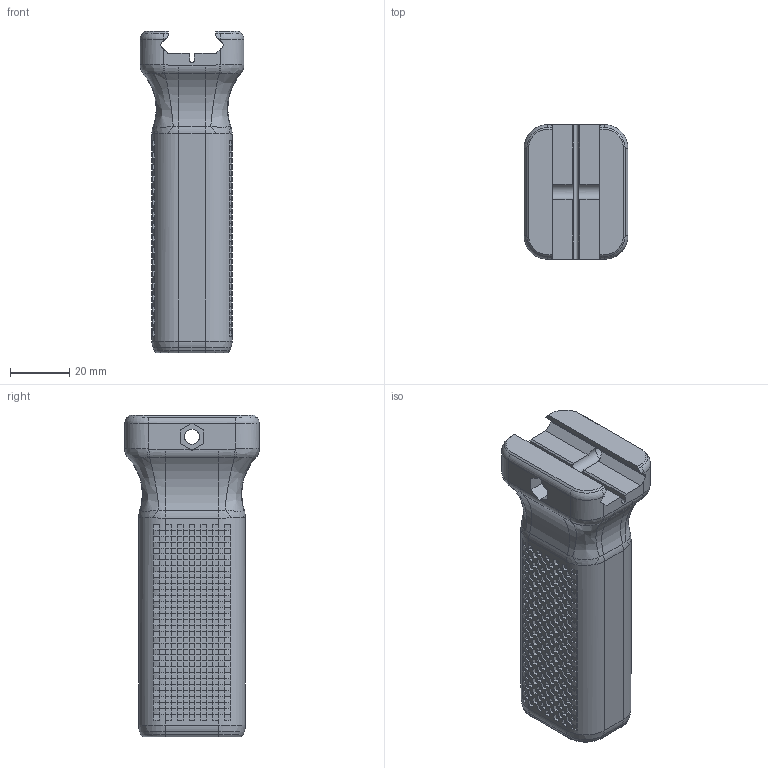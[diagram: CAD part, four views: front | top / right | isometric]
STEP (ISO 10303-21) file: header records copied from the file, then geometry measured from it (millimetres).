
FILE_DESCRIPTION(/* description */ (''),/* implementation_level */ '2;1');
FILE_NAME(/* name */ 'Checkered Model.step',/* time_stamp */ '2021-05-21T12:31:54-04:00',/* author */ (''),/* organization */ (''),/* preprocessor_version */ 'ST-DEVELOPER v18.1',/* originating_system */ 'Autodesk Translation Framework v10.6.0.1341',/* authorisation */ '');
FILE_SCHEMA (('AUTOMOTIVE_DESIGN { 1 0 10303 214 3 1 1 }'));
Products named in the file (1): Checkered Model
Bounding box: 35 x 45.3 x 108.12 mm (x, y, z)
Volume: 55236.5 mm3; surface area: 26486.5 mm2
Topology: 1 solids, 1 shells, 3015 faces, 6425 edges, 2646 vertices
Faces by surface type: plane 2725, cylinder 174, bspline 84, torus 20, cone 12
Full cylindrical faces by diameter (mm): 5.1 x2, 8.75 x1, 11.5 x1, 13 x1
Entity records: 77060 total; most frequent: CARTESIAN_POINT 14604, ORIENTED_EDGE 12842, DIRECTION 12789, EDGE_CURVE 6421, LINE 5645, VECTOR 5645, AXIS2_PLACEMENT_3D 3572, EDGE_LOOP 3025
